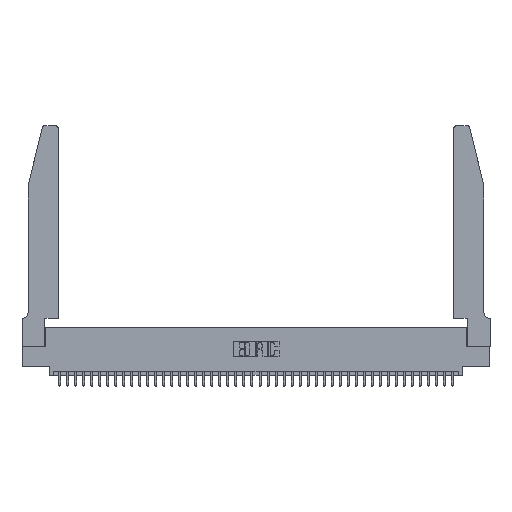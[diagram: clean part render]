
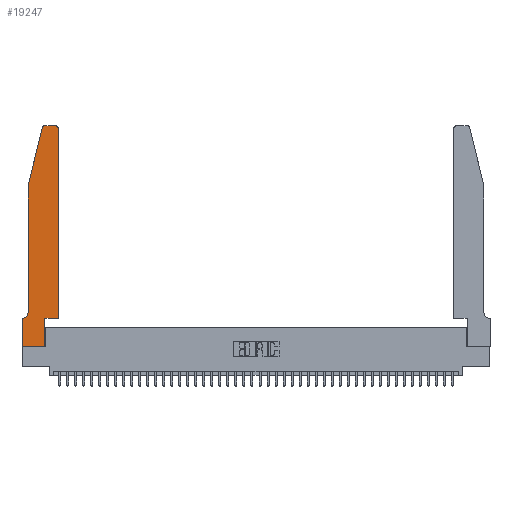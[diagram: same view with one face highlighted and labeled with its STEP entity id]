
A CAD part, top view. The second image highlights one B-rep face of the part: STEP entity #19247.
In plain terms, the highlighted planar face has unit normal (0, 0, 1).
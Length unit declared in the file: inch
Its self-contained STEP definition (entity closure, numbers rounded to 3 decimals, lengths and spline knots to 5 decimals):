
#1374 = EDGE_CURVE ( 'NONE', #11568, #32791, #36423, .T. ) ;
#1452 = VERTEX_POINT ( 'NONE', #39346 ) ;
#1663 = LINE ( 'NONE', #35253, #9540 ) ;
#2502 = ORIENTED_EDGE ( 'NONE', *, *, #42398, .T. ) ;
#3231 = CARTESIAN_POINT ( 'NONE',  ( 0.0755, 0.35, 0.37 ) ) ;
#4397 = AXIS2_PLACEMENT_3D ( 'NONE', #25971, #6037, #29308 ) ;
#4462 = EDGE_LOOP ( 'NONE', ( #10766, #29798, #9574, #32847, #9371, #19929, #37235, #21146, #36409, #27724, #23857, #2502 ) ) ;
#4971 = EDGE_CURVE ( 'NONE', #21102, #11568, #38045, .T. ) ;
#5601 = DIRECTION ( 'NONE',  ( 0., 1., 0. ) ) ;
#5872 = VECTOR ( 'NONE', #9387, 39.37008 ) ;
#5882 = DIRECTION ( 'NONE',  ( 0., -1., 0. ) ) ;
#6037 = DIRECTION ( 'NONE',  ( 0., 0., -1. ) ) ;
#6099 = LINE ( 'NONE', #32618, #31546 ) ;
#6243 = CARTESIAN_POINT ( 'NONE',  ( 0.4205, 2.72, 0.37 ) ) ;
#8583 = LINE ( 'NONE', #22191, #41814 ) ;
#8689 = VECTOR ( 'NONE', #10001, 39.37008 ) ;
#9371 = ORIENTED_EDGE ( 'NONE', *, *, #27622, .T. ) ;
#9387 = DIRECTION ( 'NONE',  ( 0., -1., 0. ) ) ;
#9540 = VECTOR ( 'NONE', #15350, 39.37008 ) ;
#9574 = ORIENTED_EDGE ( 'NONE', *, *, #15928, .T. ) ;
#9607 = DIRECTION ( 'NONE',  ( 1., 0., 0. ) ) ;
#10001 = DIRECTION ( 'NONE',  ( 1., 0., 0. ) ) ;
#10495 = VERTEX_POINT ( 'NONE', #19074 ) ;
#10766 = ORIENTED_EDGE ( 'NONE', *, *, #27294, .T. ) ;
#11270 = CARTESIAN_POINT ( 'NONE',  ( 0.2865, 0.35, 0.37 ) ) ;
#11568 = VERTEX_POINT ( 'NONE', #21270 ) ;
#11729 = CIRCLE ( 'NONE', #25421, 0.03 ) ;
#11942 = DIRECTION ( 'NONE',  ( 1., 0., 0. ) ) ;
#12506 = DIRECTION ( 'NONE',  ( 1., 0., 0. ) ) ;
#12867 = EDGE_CURVE ( 'NONE', #21231, #21102, #20623, .T. ) ;
#13469 = EDGE_CURVE ( 'NONE', #10495, #37229, #6099, .T. ) ;
#13825 = VECTOR ( 'NONE', #40869, 39.37008 ) ;
#14858 = CARTESIAN_POINT ( 'NONE',  ( 0.284, 2.72, 0.37 ) ) ;
#15350 = DIRECTION ( 'NONE',  ( -0.239, -0.971, 0. ) ) ;
#15383 = EDGE_CURVE ( 'NONE', #29034, #24931, #20472, .T. ) ;
#15928 = EDGE_CURVE ( 'NONE', #42011, #10495, #1663, .T. ) ;
#16766 = CARTESIAN_POINT ( 'NONE',  ( 0.4505, 0.35, 0.37 ) ) ;
#17863 = EDGE_CURVE ( 'NONE', #24931, #21231, #25664, .T. ) ;
#18208 = DIRECTION ( 'NONE',  ( 1., 0., 0. ) ) ;
#18275 = AXIS2_PLACEMENT_3D ( 'NONE', #28534, #38385, #11942 ) ;
#18685 = CARTESIAN_POINT ( 'NONE',  ( 0., 0., 0.37 ) ) ;
#19074 = CARTESIAN_POINT ( 'NONE',  ( 0.0755, 2., 0.37 ) ) ;
#19247 = ADVANCED_FACE ( 'NONE', ( #31200 ), #31838, .T. ) ;
#19929 = ORIENTED_EDGE ( 'NONE', *, *, #15383, .T. ) ;
#20129 = CIRCLE ( 'NONE', #20363, 0.03 ) ;
#20363 = AXIS2_PLACEMENT_3D ( 'NONE', #14858, #38090, #18208 ) ;
#20472 = LINE ( 'NONE', #3231, #37108 ) ;
#20623 = LINE ( 'NONE', #29905, #8689 ) ;
#21010 = VERTEX_POINT ( 'NONE', #37517 ) ;
#21102 = VERTEX_POINT ( 'NONE', #31409 ) ;
#21146 = ORIENTED_EDGE ( 'NONE', *, *, #12867, .T. ) ;
#21231 = VERTEX_POINT ( 'NONE', #32146 ) ;
#21270 = CARTESIAN_POINT ( 'NONE',  ( 0.2865, 0.35, 0.37 ) ) ;
#22191 = CARTESIAN_POINT ( 'NONE',  ( 0.4505, 0.35, 0.37 ) ) ;
#23669 = LINE ( 'NONE', #30882, #13825 ) ;
#23857 = ORIENTED_EDGE ( 'NONE', *, *, #31839, .T. ) ;
#24931 = VERTEX_POINT ( 'NONE', #37795 ) ;
#25421 = AXIS2_PLACEMENT_3D ( 'NONE', #6243, #29504, #9607 ) ;
#25664 = LINE ( 'NONE', #18685, #5872 ) ;
#25971 = CARTESIAN_POINT ( 'NONE',  ( 0.0055, 0.42, 0.37 ) ) ;
#26738 = CARTESIAN_POINT ( 'NONE',  ( 0.0755, 0.42, 0.37 ) ) ;
#27294 = EDGE_CURVE ( 'NONE', #41244, #1452, #23669, .T. ) ;
#27571 = VECTOR ( 'NONE', #12506, 39.37008 ) ;
#27622 = EDGE_CURVE ( 'NONE', #37229, #29034, #35651, .T. ) ;
#27724 = ORIENTED_EDGE ( 'NONE', *, *, #1374, .T. ) ;
#28534 = CARTESIAN_POINT ( 'NONE',  ( 0., 0.35, 0.37 ) ) ;
#29034 = VERTEX_POINT ( 'NONE', #40584 ) ;
#29297 = CARTESIAN_POINT ( 'NONE',  ( 0.4205, 2.75, 0.37 ) ) ;
#29308 = DIRECTION ( 'NONE',  ( -1., 0., 0. ) ) ;
#29504 = DIRECTION ( 'NONE',  ( 0., 0., 1. ) ) ;
#29798 = ORIENTED_EDGE ( 'NONE', *, *, #41690, .T. ) ;
#29905 = CARTESIAN_POINT ( 'NONE',  ( 0., 0., 0.37 ) ) ;
#30882 = CARTESIAN_POINT ( 'NONE',  ( 0.2605, 2.75, 0.37 ) ) ;
#31200 = FACE_OUTER_BOUND ( 'NONE', #4462, .T. ) ;
#31409 = CARTESIAN_POINT ( 'NONE',  ( 0.2865, 0., 0.37 ) ) ;
#31546 = VECTOR ( 'NONE', #5882, 39.37008 ) ;
#31838 = PLANE ( 'NONE',  #18275 ) ;
#31839 = EDGE_CURVE ( 'NONE', #32791, #21010, #8583, .T. ) ;
#32146 = CARTESIAN_POINT ( 'NONE',  ( 0., 0., 0.37 ) ) ;
#32618 = CARTESIAN_POINT ( 'NONE',  ( 0.0755, 2., 0.37 ) ) ;
#32791 = VERTEX_POINT ( 'NONE', #16766 ) ;
#32847 = ORIENTED_EDGE ( 'NONE', *, *, #13469, .T. ) ;
#33195 = DIRECTION ( 'NONE',  ( -1., 0., 0. ) ) ;
#34528 = DIRECTION ( 'NONE',  ( 0., 1., 0. ) ) ;
#35253 = CARTESIAN_POINT ( 'NONE',  ( 0.0755, 2., 0.37 ) ) ;
#35651 = CIRCLE ( 'NONE', #4397, 0.07 ) ;
#36369 = CARTESIAN_POINT ( 'NONE',  ( 0.25487, 2.72718, 0.37 ) ) ;
#36409 = ORIENTED_EDGE ( 'NONE', *, *, #4971, .T. ) ;
#36423 = LINE ( 'NONE', #42235, #27571 ) ;
#37108 = VECTOR ( 'NONE', #33195, 39.37008 ) ;
#37229 = VERTEX_POINT ( 'NONE', #26738 ) ;
#37235 = ORIENTED_EDGE ( 'NONE', *, *, #17863, .T. ) ;
#37517 = CARTESIAN_POINT ( 'NONE',  ( 0.4505, 2.72, 0.37 ) ) ;
#37795 = CARTESIAN_POINT ( 'NONE',  ( 0., 0.35, 0.37 ) ) ;
#38045 = LINE ( 'NONE', #11270, #39099 ) ;
#38090 = DIRECTION ( 'NONE',  ( 0., 0., 1. ) ) ;
#38385 = DIRECTION ( 'NONE',  ( 0., 0., 1. ) ) ;
#39099 = VECTOR ( 'NONE', #34528, 39.37008 ) ;
#39346 = CARTESIAN_POINT ( 'NONE',  ( 0.284, 2.75, 0.37 ) ) ;
#40584 = CARTESIAN_POINT ( 'NONE',  ( 0.0055, 0.35, 0.37 ) ) ;
#40869 = DIRECTION ( 'NONE',  ( -1., 0., 0. ) ) ;
#41244 = VERTEX_POINT ( 'NONE', #29297 ) ;
#41690 = EDGE_CURVE ( 'NONE', #1452, #42011, #20129, .T. ) ;
#41814 = VECTOR ( 'NONE', #5601, 39.37008 ) ;
#42011 = VERTEX_POINT ( 'NONE', #36369 ) ;
#42235 = CARTESIAN_POINT ( 'NONE',  ( 0.4505, 0.35, 0.37 ) ) ;
#42398 = EDGE_CURVE ( 'NONE', #21010, #41244, #11729, .T. ) ;
